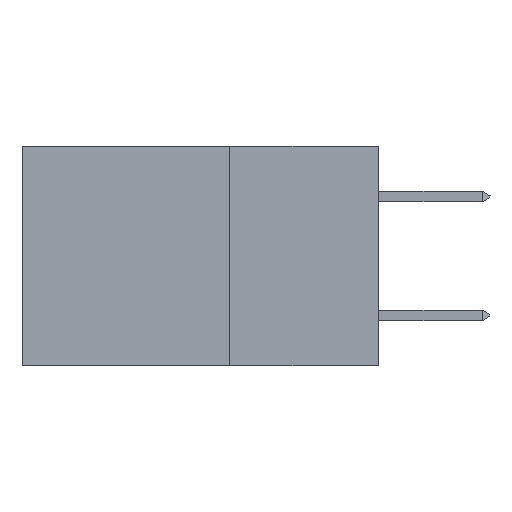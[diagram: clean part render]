
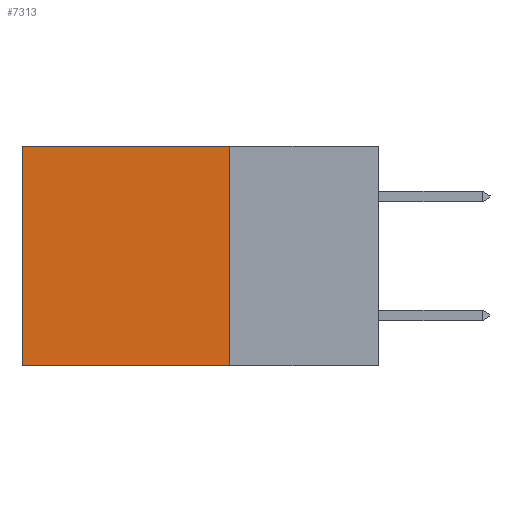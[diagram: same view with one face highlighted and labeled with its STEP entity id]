
A CAD part, left-side view. The second image highlights one B-rep face of the part: STEP entity #7313.
In plain terms, the highlighted planar face has unit normal (-1, 0, 0).
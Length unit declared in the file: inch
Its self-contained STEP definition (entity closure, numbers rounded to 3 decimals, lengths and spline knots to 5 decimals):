
#146 = VERTEX_POINT ( 'NONE', #4928 ) ;
#301 = DIRECTION ( 'NONE',  ( 1., 0., 0. ) ) ;
#731 = VECTOR ( 'NONE', #1107, 39.37008 ) ;
#750 = VECTOR ( 'NONE', #3962, 39.37008 ) ;
#1107 = DIRECTION ( 'NONE',  ( 0., 0., -1. ) ) ;
#1871 = PLANE ( 'NONE',  #9527 ) ;
#2062 = VERTEX_POINT ( 'NONE', #5284 ) ;
#2535 = EDGE_CURVE ( 'NONE', #2720, #2062, #8954, .T. ) ;
#2563 = CARTESIAN_POINT ( 'NONE',  ( 0.2615, 0.25, -0.37 ) ) ;
#2720 = VERTEX_POINT ( 'NONE', #7496 ) ;
#2739 = CARTESIAN_POINT ( 'NONE',  ( 0.2615, 0.25, -0.37 ) ) ;
#2892 = EDGE_LOOP ( 'NONE', ( #4105, #4602, #5239, #10217 ) ) ;
#2894 = VECTOR ( 'NONE', #10442, 39.37008 ) ;
#3389 = CARTESIAN_POINT ( 'NONE',  ( 0.2615, 0.25, 0. ) ) ;
#3580 = DIRECTION ( 'NONE',  ( 0., 0., -1. ) ) ;
#3740 = CARTESIAN_POINT ( 'NONE',  ( 0.2615, 0.25, -0.37 ) ) ;
#3859 = VERTEX_POINT ( 'NONE', #3740 ) ;
#3962 = DIRECTION ( 'NONE',  ( 0., 1., 0. ) ) ;
#4105 = ORIENTED_EDGE ( 'NONE', *, *, #2535, .T. ) ;
#4602 = ORIENTED_EDGE ( 'NONE', *, *, #9990, .F. ) ;
#4928 = CARTESIAN_POINT ( 'NONE',  ( 0.2615, 0.25, 0. ) ) ;
#5239 = ORIENTED_EDGE ( 'NONE', *, *, #10692, .F. ) ;
#5284 = CARTESIAN_POINT ( 'NONE',  ( 0.2615, 0.6, -0.37 ) ) ;
#5860 = LINE ( 'NONE', #9746, #750 ) ;
#6078 = VECTOR ( 'NONE', #6681, 39.37008 ) ;
#6330 = EDGE_CURVE ( 'NONE', #146, #2720, #7493, .T. ) ;
#6681 = DIRECTION ( 'NONE',  ( 0., 1., 0. ) ) ;
#7313 = ADVANCED_FACE ( 'NONE', ( #9466 ), #1871, .F. ) ;
#7493 = LINE ( 'NONE', #3389, #6078 ) ;
#7496 = CARTESIAN_POINT ( 'NONE',  ( 0.2615, 0.6, 0. ) ) ;
#8404 = LINE ( 'NONE', #2563, #731 ) ;
#8954 = LINE ( 'NONE', #9011, #2894 ) ;
#9011 = CARTESIAN_POINT ( 'NONE',  ( 0.2615, 0.6, -0.37 ) ) ;
#9466 = FACE_OUTER_BOUND ( 'NONE', #2892, .T. ) ;
#9527 = AXIS2_PLACEMENT_3D ( 'NONE', #2739, #301, #3580 ) ;
#9746 = CARTESIAN_POINT ( 'NONE',  ( 0.2615, 0.25, -0.37 ) ) ;
#9990 = EDGE_CURVE ( 'NONE', #3859, #2062, #5860, .T. ) ;
#10217 = ORIENTED_EDGE ( 'NONE', *, *, #6330, .T. ) ;
#10442 = DIRECTION ( 'NONE',  ( 0., 0., -1. ) ) ;
#10692 = EDGE_CURVE ( 'NONE', #146, #3859, #8404, .T. ) ;
